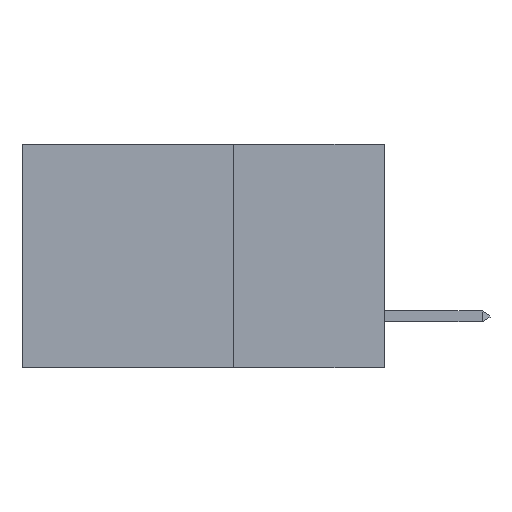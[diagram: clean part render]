
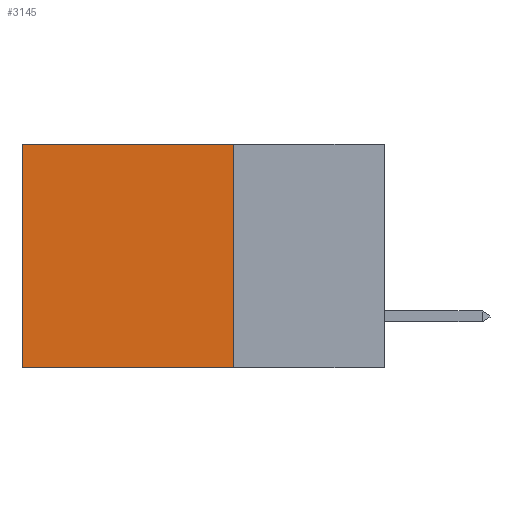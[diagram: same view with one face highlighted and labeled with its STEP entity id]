
A CAD part, left-side view. The second image highlights one B-rep face of the part: STEP entity #3145.
In plain terms, the highlighted planar face has unit normal (-1, 0, 0).
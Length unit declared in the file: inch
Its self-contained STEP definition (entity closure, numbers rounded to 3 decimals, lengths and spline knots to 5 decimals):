
#1652 = CARTESIAN_POINT ( 'NONE',  ( 0.2875, 0.25, -0.37 ) ) ;
#1710 = VERTEX_POINT ( 'NONE', #14976 ) ;
#3145 = ADVANCED_FACE ( 'NONE', ( #22512 ), #20357, .F. ) ;
#3254 = EDGE_CURVE ( 'NONE', #8628, #1710, #20292, .T. ) ;
#4172 = VECTOR ( 'NONE', #14764, 39.37008 ) ;
#6310 = CARTESIAN_POINT ( 'NONE',  ( 0.2875, 0.6, 0. ) ) ;
#6324 = LINE ( 'NONE', #1652, #20275 ) ;
#7902 = CARTESIAN_POINT ( 'NONE',  ( 0.2875, 0.6, 0. ) ) ;
#8628 = VERTEX_POINT ( 'NONE', #16613 ) ;
#10503 = VECTOR ( 'NONE', #20602, 39.37008 ) ;
#10627 = EDGE_CURVE ( 'NONE', #13346, #20685, #14751, .T. ) ;
#11382 = DIRECTION ( 'NONE',  ( 0., 0., -1. ) ) ;
#12466 = ORIENTED_EDGE ( 'NONE', *, *, #12991, .F. ) ;
#12705 = DIRECTION ( 'NONE',  ( 0., 1., 0. ) ) ;
#12991 = EDGE_CURVE ( 'NONE', #1710, #20685, #6324, .T. ) ;
#13346 = VERTEX_POINT ( 'NONE', #6310 ) ;
#13510 = DIRECTION ( 'NONE',  ( 0., 0., -1. ) ) ;
#14646 = ORIENTED_EDGE ( 'NONE', *, *, #3254, .F. ) ;
#14751 = LINE ( 'NONE', #7902, #10503 ) ;
#14764 = DIRECTION ( 'NONE',  ( 0., 1., 0. ) ) ;
#14909 = CARTESIAN_POINT ( 'NONE',  ( 0.2875, 0.6, -0.37 ) ) ;
#14976 = CARTESIAN_POINT ( 'NONE',  ( 0.2875, 0.25, -0.37 ) ) ;
#15508 = VECTOR ( 'NONE', #13510, 39.37008 ) ;
#16188 = ORIENTED_EDGE ( 'NONE', *, *, #18598, .T. ) ;
#16613 = CARTESIAN_POINT ( 'NONE',  ( 0.2875, 0.25, 0. ) ) ;
#18137 = AXIS2_PLACEMENT_3D ( 'NONE', #19960, #22146, #11382 ) ;
#18424 = CARTESIAN_POINT ( 'NONE',  ( 0.2875, 0.25, 0. ) ) ;
#18598 = EDGE_CURVE ( 'NONE', #8628, #13346, #23430, .T. ) ;
#19960 = CARTESIAN_POINT ( 'NONE',  ( 0.2875, 0.25, 0. ) ) ;
#20275 = VECTOR ( 'NONE', #12705, 39.37008 ) ;
#20292 = LINE ( 'NONE', #20663, #15508 ) ;
#20357 = PLANE ( 'NONE',  #18137 ) ;
#20592 = ORIENTED_EDGE ( 'NONE', *, *, #10627, .T. ) ;
#20602 = DIRECTION ( 'NONE',  ( 0., 0., -1. ) ) ;
#20663 = CARTESIAN_POINT ( 'NONE',  ( 0.2875, 0.25, 0. ) ) ;
#20685 = VERTEX_POINT ( 'NONE', #14909 ) ;
#21467 = EDGE_LOOP ( 'NONE', ( #20592, #12466, #14646, #16188 ) ) ;
#22146 = DIRECTION ( 'NONE',  ( 1., 0., 0. ) ) ;
#22512 = FACE_OUTER_BOUND ( 'NONE', #21467, .T. ) ;
#23430 = LINE ( 'NONE', #18424, #4172 ) ;
